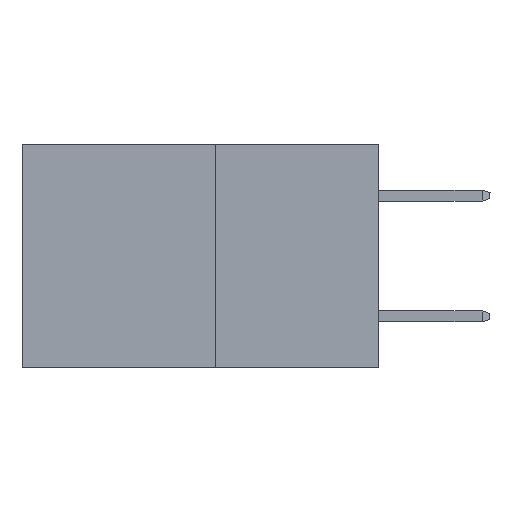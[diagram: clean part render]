
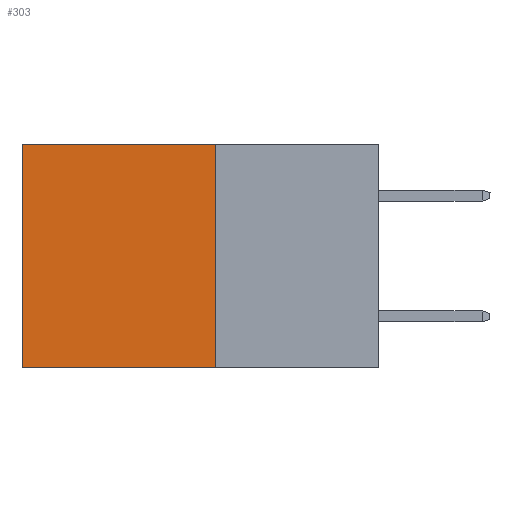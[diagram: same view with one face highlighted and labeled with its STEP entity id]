
A CAD part, left-side view. The second image highlights one B-rep face of the part: STEP entity #303.
In plain terms, the highlighted planar face has unit normal (-1, 0, 0).
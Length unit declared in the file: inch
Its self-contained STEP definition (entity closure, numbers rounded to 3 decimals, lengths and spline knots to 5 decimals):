
#303 = ADVANCED_FACE ( 'NONE', ( #1026 ), #2212, .F. ) ;
#415 = DIRECTION ( 'NONE',  ( 0., 0., -1. ) ) ;
#1026 = FACE_OUTER_BOUND ( 'NONE', #4104, .T. ) ;
#1700 = DIRECTION ( 'NONE',  ( 0., 1., 0. ) ) ;
#2083 = EDGE_CURVE ( 'NONE', #7752, #2122, #7267, .T. ) ;
#2122 = VERTEX_POINT ( 'NONE', #6528 ) ;
#2136 = ORIENTED_EDGE ( 'NONE', *, *, #8862, .F. ) ;
#2212 = PLANE ( 'NONE',  #2943 ) ;
#2354 = ORIENTED_EDGE ( 'NONE', *, *, #2572, .T. ) ;
#2362 = VECTOR ( 'NONE', #3124, 39.37008 ) ;
#2373 = VERTEX_POINT ( 'NONE', #6180 ) ;
#2572 = EDGE_CURVE ( 'NONE', #8807, #7752, #5228, .T. ) ;
#2943 = AXIS2_PLACEMENT_3D ( 'NONE', #9108, #3928, #4866 ) ;
#3094 = CARTESIAN_POINT ( 'NONE',  ( 0.277, 0.27, -0.37 ) ) ;
#3124 = DIRECTION ( 'NONE',  ( 0., 0., -1. ) ) ;
#3428 = DIRECTION ( 'NONE',  ( 0., 1., 0. ) ) ;
#3498 = CARTESIAN_POINT ( 'NONE',  ( 0.277, 0.27, 0. ) ) ;
#3928 = DIRECTION ( 'NONE',  ( 1., 0., 0. ) ) ;
#4104 = EDGE_LOOP ( 'NONE', ( #7432, #2136, #7652, #2354 ) ) ;
#4477 = CARTESIAN_POINT ( 'NONE',  ( 0.277, 0.27, -0.37 ) ) ;
#4866 = DIRECTION ( 'NONE',  ( 0., 0., -1. ) ) ;
#5228 = LINE ( 'NONE', #3498, #8655 ) ;
#6036 = LINE ( 'NONE', #3094, #2362 ) ;
#6180 = CARTESIAN_POINT ( 'NONE',  ( 0.277, 0.27, -0.37 ) ) ;
#6271 = CARTESIAN_POINT ( 'NONE',  ( 0.277, 0.59, 0. ) ) ;
#6528 = CARTESIAN_POINT ( 'NONE',  ( 0.277, 0.59, -0.37 ) ) ;
#7267 = LINE ( 'NONE', #8220, #7713 ) ;
#7432 = ORIENTED_EDGE ( 'NONE', *, *, #2083, .T. ) ;
#7652 = ORIENTED_EDGE ( 'NONE', *, *, #8887, .F. ) ;
#7713 = VECTOR ( 'NONE', #415, 39.37008 ) ;
#7752 = VERTEX_POINT ( 'NONE', #6271 ) ;
#7869 = VECTOR ( 'NONE', #1700, 39.37008 ) ;
#8220 = CARTESIAN_POINT ( 'NONE',  ( 0.277, 0.59, -0.37 ) ) ;
#8301 = LINE ( 'NONE', #4477, #7869 ) ;
#8545 = CARTESIAN_POINT ( 'NONE',  ( 0.277, 0.27, 0. ) ) ;
#8655 = VECTOR ( 'NONE', #3428, 39.37008 ) ;
#8807 = VERTEX_POINT ( 'NONE', #8545 ) ;
#8862 = EDGE_CURVE ( 'NONE', #2373, #2122, #8301, .T. ) ;
#8887 = EDGE_CURVE ( 'NONE', #8807, #2373, #6036, .T. ) ;
#9108 = CARTESIAN_POINT ( 'NONE',  ( 0.277, 0.27, -0.37 ) ) ;
